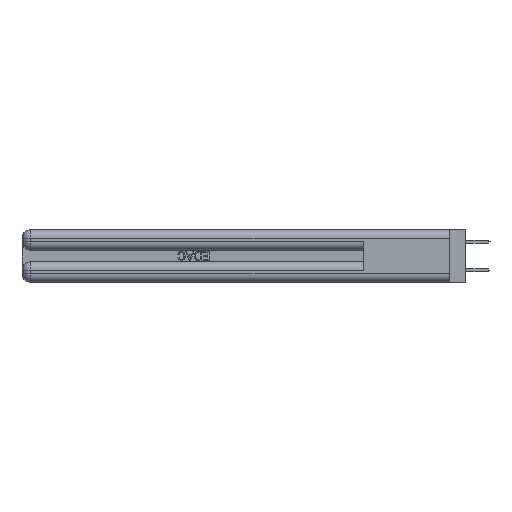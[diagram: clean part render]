
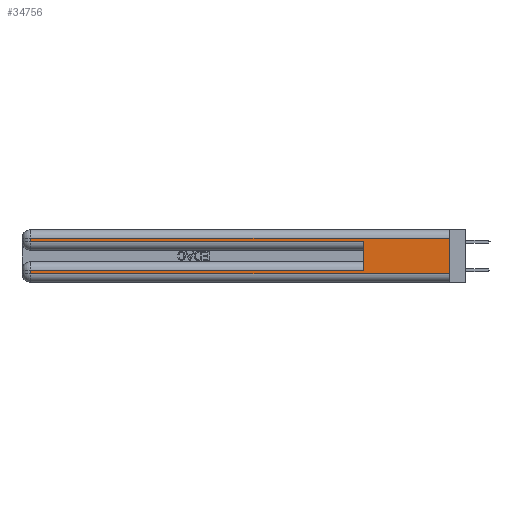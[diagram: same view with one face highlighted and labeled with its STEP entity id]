
A CAD part, left-side view. The second image highlights one B-rep face of the part: STEP entity #34756.
In plain terms, the highlighted planar face has unit normal (-1, 0, 0).
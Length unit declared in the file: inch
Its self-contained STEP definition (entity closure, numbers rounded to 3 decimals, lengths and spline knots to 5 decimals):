
#655 = VERTEX_POINT ( 'NONE', #31184 ) ;
#848 = LINE ( 'NONE', #36879, #19738 ) ;
#1597 = CARTESIAN_POINT ( 'NONE',  ( 0., 2.94, 0.085 ) ) ;
#2398 = AXIS2_PLACEMENT_3D ( 'NONE', #29458, #29183, #38505 ) ;
#2474 = LINE ( 'NONE', #37192, #24768 ) ;
#3214 = VERTEX_POINT ( 'NONE', #30819 ) ;
#3664 = VERTEX_POINT ( 'NONE', #30061 ) ;
#3771 = EDGE_CURVE ( 'NONE', #3214, #655, #848, .T. ) ;
#4471 = EDGE_CURVE ( 'NONE', #655, #12825, #14280, .T. ) ;
#5208 = CARTESIAN_POINT ( 'NONE',  ( 0., 0., 0.37 ) ) ;
#5271 = CARTESIAN_POINT ( 'NONE',  ( 0., 2.94, 0.06 ) ) ;
#7648 = VERTEX_POINT ( 'NONE', #31015 ) ;
#7939 = DIRECTION ( 'NONE',  ( 0., 1., 0. ) ) ;
#10141 = DIRECTION ( 'NONE',  ( 0., 0., 1. ) ) ;
#10800 = ORIENTED_EDGE ( 'NONE', *, *, #4471, .T. ) ;
#11214 = VECTOR ( 'NONE', #17968, 39.37008 ) ;
#12042 = ORIENTED_EDGE ( 'NONE', *, *, #12437, .F. ) ;
#12437 = EDGE_CURVE ( 'NONE', #16153, #3664, #37798, .T. ) ;
#12825 = VERTEX_POINT ( 'NONE', #25158 ) ;
#13437 = ORIENTED_EDGE ( 'NONE', *, *, #3771, .T. ) ;
#13492 = CARTESIAN_POINT ( 'NONE',  ( 0., 0., 0.285 ) ) ;
#14280 = LINE ( 'NONE', #13492, #27647 ) ;
#14371 = DIRECTION ( 'NONE',  ( 0., 0., -1. ) ) ;
#14614 = CARTESIAN_POINT ( 'NONE',  ( 0., 0., 0.31 ) ) ;
#15054 = CARTESIAN_POINT ( 'NONE',  ( 0., 0., 0.06 ) ) ;
#15943 = VERTEX_POINT ( 'NONE', #5271 ) ;
#16108 = VECTOR ( 'NONE', #19638, 39.37008 ) ;
#16153 = VERTEX_POINT ( 'NONE', #28401 ) ;
#16418 = PLANE ( 'NONE',  #2398 ) ;
#16799 = DIRECTION ( 'NONE',  ( 0., -1., 0. ) ) ;
#16871 = FACE_OUTER_BOUND ( 'NONE', #29764, .T. ) ;
#17968 = DIRECTION ( 'NONE',  ( 0., -1., 0. ) ) ;
#18299 = DIRECTION ( 'NONE',  ( 0., 0., -1. ) ) ;
#18567 = VECTOR ( 'NONE', #21275, 39.37008 ) ;
#18645 = VECTOR ( 'NONE', #10141, 39.37008 ) ;
#18994 = VERTEX_POINT ( 'NONE', #1597 ) ;
#19629 = LINE ( 'NONE', #15054, #11214 ) ;
#19638 = DIRECTION ( 'NONE',  ( 0., 1., 0. ) ) ;
#19738 = VECTOR ( 'NONE', #14371, 39.37008 ) ;
#20373 = VECTOR ( 'NONE', #7939, 39.37008 ) ;
#21275 = DIRECTION ( 'NONE',  ( 0., 0., -1. ) ) ;
#24562 = LINE ( 'NONE', #29482, #16108 ) ;
#24768 = VECTOR ( 'NONE', #18299, 39.37008 ) ;
#25158 = CARTESIAN_POINT ( 'NONE',  ( 0., 0.6, 0.285 ) ) ;
#25474 = ORIENTED_EDGE ( 'NONE', *, *, #40887, .T. ) ;
#25934 = CARTESIAN_POINT ( 'NONE',  ( 0., 0.6, 0.145 ) ) ;
#27647 = VECTOR ( 'NONE', #16799, 39.37008 ) ;
#28401 = CARTESIAN_POINT ( 'NONE',  ( 0., 0., 0.31 ) ) ;
#28550 = LINE ( 'NONE', #25934, #18645 ) ;
#28915 = ORIENTED_EDGE ( 'NONE', *, *, #36309, .T. ) ;
#28979 = ORIENTED_EDGE ( 'NONE', *, *, #37980, .F. ) ;
#29183 = DIRECTION ( 'NONE',  ( 1., 0., 0. ) ) ;
#29458 = CARTESIAN_POINT ( 'NONE',  ( 0., 0., 0.37 ) ) ;
#29482 = CARTESIAN_POINT ( 'NONE',  ( 0., 0., 0.085 ) ) ;
#29568 = ORIENTED_EDGE ( 'NONE', *, *, #33701, .T. ) ;
#29764 = EDGE_LOOP ( 'NONE', ( #12042, #40740, #13437, #10800, #28979, #25474, #28915, #29568 ) ) ;
#30061 = CARTESIAN_POINT ( 'NONE',  ( 0., 0., 0.06 ) ) ;
#30819 = CARTESIAN_POINT ( 'NONE',  ( 0., 2.94, 0.31 ) ) ;
#31015 = CARTESIAN_POINT ( 'NONE',  ( 0., 0.6, 0.085 ) ) ;
#31184 = CARTESIAN_POINT ( 'NONE',  ( 0., 2.94, 0.285 ) ) ;
#31253 = EDGE_CURVE ( 'NONE', #16153, #3214, #33711, .T. ) ;
#33701 = EDGE_CURVE ( 'NONE', #15943, #3664, #19629, .T. ) ;
#33711 = LINE ( 'NONE', #14614, #20373 ) ;
#34756 = ADVANCED_FACE ( 'NONE', ( #16871 ), #16418, .F. ) ;
#36309 = EDGE_CURVE ( 'NONE', #18994, #15943, #2474, .T. ) ;
#36879 = CARTESIAN_POINT ( 'NONE',  ( 0., 2.94, 0.37 ) ) ;
#37192 = CARTESIAN_POINT ( 'NONE',  ( 0., 2.94, 0.37 ) ) ;
#37798 = LINE ( 'NONE', #5208, #18567 ) ;
#37980 = EDGE_CURVE ( 'NONE', #7648, #12825, #28550, .T. ) ;
#38505 = DIRECTION ( 'NONE',  ( 0., 0., -1. ) ) ;
#40740 = ORIENTED_EDGE ( 'NONE', *, *, #31253, .T. ) ;
#40887 = EDGE_CURVE ( 'NONE', #7648, #18994, #24562, .T. ) ;
